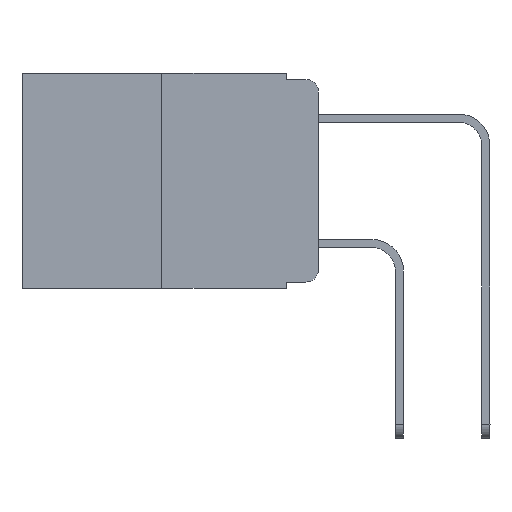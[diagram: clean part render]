
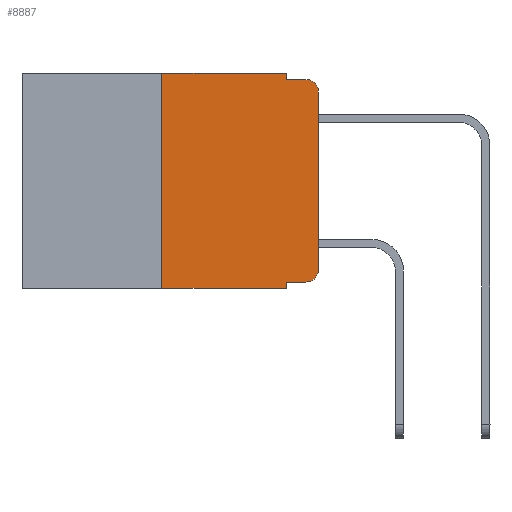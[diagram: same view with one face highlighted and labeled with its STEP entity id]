
A CAD part, left-side view. The second image highlights one B-rep face of the part: STEP entity #8887.
In plain terms, the highlighted planar face has unit normal (-1, 0, 0).
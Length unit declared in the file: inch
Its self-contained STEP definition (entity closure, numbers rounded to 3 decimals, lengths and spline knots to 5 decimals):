
#918 = ORIENTED_EDGE ( 'NONE', *, *, #17817, .F. ) ;
#1351 = AXIS2_PLACEMENT_3D ( 'NONE', #15387, #2432, #9537 ) ;
#1618 = DIRECTION ( 'NONE',  ( -1., 0., 0. ) ) ;
#1795 = DIRECTION ( 'NONE',  ( 0., 0., -1. ) ) ;
#2013 = LINE ( 'NONE', #9002, #12062 ) ;
#2432 = DIRECTION ( 'NONE',  ( 1., 0., 0. ) ) ;
#3143 = CARTESIAN_POINT ( 'NONE',  ( 0., 0., -0.03 ) ) ;
#3231 = LINE ( 'NONE', #8917, #7246 ) ;
#3353 = VERTEX_POINT ( 'NONE', #13289 ) ;
#3422 = DIRECTION ( 'NONE',  ( 0., 0., 1. ) ) ;
#3808 = CARTESIAN_POINT ( 'NONE',  ( 0., 0.473, 0. ) ) ;
#3967 = AXIS2_PLACEMENT_3D ( 'NONE', #4093, #8385, #9703 ) ;
#4093 = CARTESIAN_POINT ( 'NONE',  ( 0., 0.02, -0.03 ) ) ;
#4558 = LINE ( 'NONE', #14092, #6020 ) ;
#4568 = EDGE_CURVE ( 'NONE', #6664, #10982, #4558, .T. ) ;
#4748 = EDGE_CURVE ( 'NONE', #11419, #3353, #6041, .T. ) ;
#4867 = EDGE_CURVE ( 'NONE', #8171, #3353, #6029, .T. ) ;
#5162 = EDGE_CURVE ( 'NONE', #10701, #8171, #3231, .T. ) ;
#5224 = CARTESIAN_POINT ( 'NONE',  ( 0., 0.25, 0. ) ) ;
#5950 = VERTEX_POINT ( 'NONE', #12599 ) ;
#6020 = VECTOR ( 'NONE', #11172, 39.37008 ) ;
#6029 = CIRCLE ( 'NONE', #3967, 0.02 ) ;
#6041 = LINE ( 'NONE', #13293, #13552 ) ;
#6092 = ORIENTED_EDGE ( 'NONE', *, *, #17198, .F. ) ;
#6664 = VERTEX_POINT ( 'NONE', #8264 ) ;
#6781 = CARTESIAN_POINT ( 'NONE',  ( 0., 0.051, -0.333 ) ) ;
#6808 = LINE ( 'NONE', #18297, #10516 ) ;
#6900 = EDGE_LOOP ( 'NONE', ( #18461, #12566, #15084, #918, #18007, #15295, #11342, #6092, #15677, #13642 ) ) ;
#7093 = CARTESIAN_POINT ( 'NONE',  ( 0., 0.051, -0.01 ) ) ;
#7246 = VECTOR ( 'NONE', #3422, 39.37008 ) ;
#8030 = FACE_OUTER_BOUND ( 'NONE', #6900, .T. ) ;
#8171 = VERTEX_POINT ( 'NONE', #3143 ) ;
#8264 = CARTESIAN_POINT ( 'NONE',  ( 0., 0.25, -0.343 ) ) ;
#8385 = DIRECTION ( 'NONE',  ( -1., 0., 0. ) ) ;
#8887 = ADVANCED_FACE ( 'NONE', ( #8030 ), #12483, .F. ) ;
#8917 = CARTESIAN_POINT ( 'NONE',  ( 0., 0., 0. ) ) ;
#9002 = CARTESIAN_POINT ( 'NONE',  ( 0., 0.051, 0. ) ) ;
#9204 = DIRECTION ( 'NONE',  ( 0., 0., 1. ) ) ;
#9215 = CARTESIAN_POINT ( 'NONE',  ( 0., 0., -0.313 ) ) ;
#9434 = LINE ( 'NONE', #3808, #18068 ) ;
#9537 = DIRECTION ( 'NONE',  ( 0., 0., -1. ) ) ;
#9703 = DIRECTION ( 'NONE',  ( 0., 0., -1. ) ) ;
#10236 = DIRECTION ( 'NONE',  ( 0., 0., -1. ) ) ;
#10288 = CARTESIAN_POINT ( 'NONE',  ( 0., 0.051, -0.333 ) ) ;
#10470 = EDGE_CURVE ( 'NONE', #11677, #5950, #9434, .T. ) ;
#10516 = VECTOR ( 'NONE', #15099, 39.37008 ) ;
#10701 = VERTEX_POINT ( 'NONE', #9215 ) ;
#10714 = LINE ( 'NONE', #18152, #16547 ) ;
#10925 = CARTESIAN_POINT ( 'NONE',  ( 0., 0.051, -0.343 ) ) ;
#10982 = VERTEX_POINT ( 'NONE', #10925 ) ;
#11172 = DIRECTION ( 'NONE',  ( 0., -1., 0. ) ) ;
#11342 = ORIENTED_EDGE ( 'NONE', *, *, #4568, .T. ) ;
#11419 = VERTEX_POINT ( 'NONE', #7093 ) ;
#11677 = VERTEX_POINT ( 'NONE', #5224 ) ;
#11788 = DIRECTION ( 'NONE',  ( 0., -1., 0. ) ) ;
#12062 = VECTOR ( 'NONE', #10236, 39.37008 ) ;
#12150 = VERTEX_POINT ( 'NONE', #6781 ) ;
#12460 = DIRECTION ( 'NONE',  ( 0., -1., 0. ) ) ;
#12483 = PLANE ( 'NONE',  #1351 ) ;
#12566 = ORIENTED_EDGE ( 'NONE', *, *, #4867, .T. ) ;
#12599 = CARTESIAN_POINT ( 'NONE',  ( 0., 0.051, 0. ) ) ;
#13289 = CARTESIAN_POINT ( 'NONE',  ( 0., 0.02, -0.01 ) ) ;
#13293 = CARTESIAN_POINT ( 'NONE',  ( 0., 0.051, -0.01 ) ) ;
#13552 = VECTOR ( 'NONE', #11788, 39.37008 ) ;
#13642 = ORIENTED_EDGE ( 'NONE', *, *, #18338, .T. ) ;
#14092 = CARTESIAN_POINT ( 'NONE',  ( 0., 0.473, -0.343 ) ) ;
#14463 = CARTESIAN_POINT ( 'NONE',  ( 0., 0.02, -0.313 ) ) ;
#14540 = VERTEX_POINT ( 'NONE', #16685 ) ;
#14752 = VECTOR ( 'NONE', #16041, 39.37008 ) ;
#14773 = CIRCLE ( 'NONE', #18071, 0.02 ) ;
#15084 = ORIENTED_EDGE ( 'NONE', *, *, #4748, .F. ) ;
#15099 = DIRECTION ( 'NONE',  ( 0., 0., -1. ) ) ;
#15295 = ORIENTED_EDGE ( 'NONE', *, *, #18023, .F. ) ;
#15387 = CARTESIAN_POINT ( 'NONE',  ( 0., 0.473, 0. ) ) ;
#15633 = EDGE_CURVE ( 'NONE', #12150, #14540, #17543, .T. ) ;
#15677 = ORIENTED_EDGE ( 'NONE', *, *, #15633, .T. ) ;
#16041 = DIRECTION ( 'NONE',  ( 0., -1., 0. ) ) ;
#16547 = VECTOR ( 'NONE', #9204, 39.37008 ) ;
#16685 = CARTESIAN_POINT ( 'NONE',  ( 0., 0.02, -0.333 ) ) ;
#17198 = EDGE_CURVE ( 'NONE', #12150, #10982, #6808, .T. ) ;
#17543 = LINE ( 'NONE', #10288, #14752 ) ;
#17817 = EDGE_CURVE ( 'NONE', #5950, #11419, #2013, .T. ) ;
#18007 = ORIENTED_EDGE ( 'NONE', *, *, #10470, .F. ) ;
#18023 = EDGE_CURVE ( 'NONE', #6664, #11677, #10714, .T. ) ;
#18068 = VECTOR ( 'NONE', #12460, 39.37008 ) ;
#18071 = AXIS2_PLACEMENT_3D ( 'NONE', #14463, #1618, #1795 ) ;
#18152 = CARTESIAN_POINT ( 'NONE',  ( 0., 0.25, 0. ) ) ;
#18297 = CARTESIAN_POINT ( 'NONE',  ( 0., 0.051, 0. ) ) ;
#18338 = EDGE_CURVE ( 'NONE', #14540, #10701, #14773, .T. ) ;
#18461 = ORIENTED_EDGE ( 'NONE', *, *, #5162, .T. ) ;
